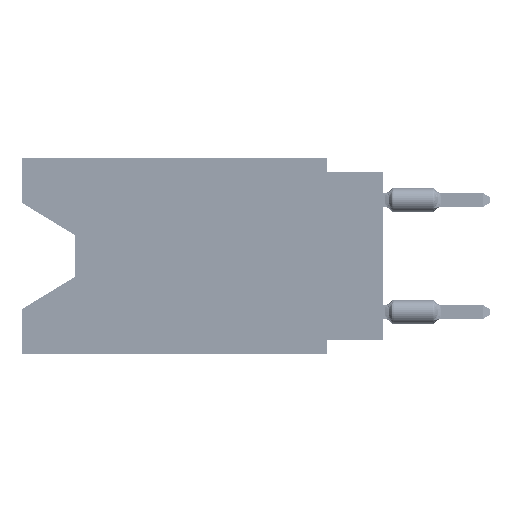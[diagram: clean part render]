
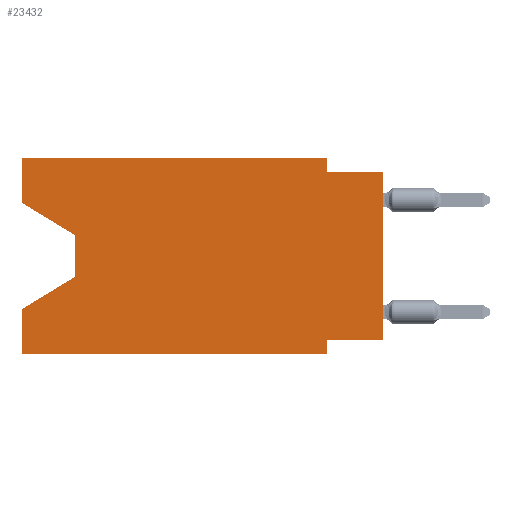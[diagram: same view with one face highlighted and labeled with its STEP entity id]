
A CAD part, left-side view. The second image highlights one B-rep face of the part: STEP entity #23432.
In plain terms, the highlighted planar face has unit normal (-1, 0, 0).
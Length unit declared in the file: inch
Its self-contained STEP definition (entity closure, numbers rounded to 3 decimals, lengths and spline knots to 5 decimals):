
#616 = EDGE_CURVE ( 'NONE', #29009, #13875, #54126, .T. ) ;
#1724 = VECTOR ( 'NONE', #10512, 39.37008 ) ;
#2000 = CARTESIAN_POINT ( 'NONE',  ( 0., 0.1, 0. ) ) ;
#3656 = CARTESIAN_POINT ( 'NONE',  ( 0., 0.645, -0.26975 ) ) ;
#3871 = LINE ( 'NONE', #20720, #44310 ) ;
#3898 = CARTESIAN_POINT ( 'NONE',  ( 0., 0.1, 0. ) ) ;
#3930 = DIRECTION ( 'NONE',  ( 0., 1., 0. ) ) ;
#5901 = LINE ( 'NONE', #15821, #15807 ) ;
#6034 = DIRECTION ( 'NONE',  ( 0., -1., 0. ) ) ;
#6709 = CARTESIAN_POINT ( 'NONE',  ( 0., 0.55, -0.212 ) ) ;
#7014 = EDGE_CURVE ( 'NONE', #55235, #61821, #58415, .T. ) ;
#7675 = EDGE_CURVE ( 'NONE', #13875, #41816, #28992, .T. ) ;
#8223 = DIRECTION ( 'NONE',  ( 0., 0., -1. ) ) ;
#9641 = EDGE_CURVE ( 'NONE', #24184, #34143, #23411, .T. ) ;
#10512 = DIRECTION ( 'NONE',  ( 0., 0., 1. ) ) ;
#11020 = ORIENTED_EDGE ( 'NONE', *, *, #616, .F. ) ;
#12656 = EDGE_CURVE ( 'NONE', #18530, #20161, #29989, .T. ) ;
#13194 = CARTESIAN_POINT ( 'NONE',  ( 0., 0.645, -0.35 ) ) ;
#13875 = VERTEX_POINT ( 'NONE', #60011 ) ;
#13877 = VERTEX_POINT ( 'NONE', #15309 ) ;
#14390 = CARTESIAN_POINT ( 'NONE',  ( 0., 0.1, -0.025 ) ) ;
#15309 = CARTESIAN_POINT ( 'NONE',  ( 0., 0.645, -0.35 ) ) ;
#15742 = EDGE_CURVE ( 'NONE', #61821, #40443, #40611, .T. ) ;
#15807 = VECTOR ( 'NONE', #71864, 39.37008 ) ;
#15821 = CARTESIAN_POINT ( 'NONE',  ( 0., 0.55, -0.212 ) ) ;
#16008 = LINE ( 'NONE', #44210, #1724 ) ;
#17539 = ORIENTED_EDGE ( 'NONE', *, *, #7014, .F. ) ;
#18102 = VECTOR ( 'NONE', #24503, 39.37008 ) ;
#18242 = CARTESIAN_POINT ( 'NONE',  ( 0., 0., -0.025 ) ) ;
#18431 = ORIENTED_EDGE ( 'NONE', *, *, #35811, .T. ) ;
#18530 = VERTEX_POINT ( 'NONE', #44497 ) ;
#19675 = CARTESIAN_POINT ( 'NONE',  ( 0., 0.645, -0.08025 ) ) ;
#20161 = VERTEX_POINT ( 'NONE', #50193 ) ;
#20720 = CARTESIAN_POINT ( 'NONE',  ( 0., 0.645, 0. ) ) ;
#21095 = ORIENTED_EDGE ( 'NONE', *, *, #34556, .T. ) ;
#22560 = ORIENTED_EDGE ( 'NONE', *, *, #15742, .F. ) ;
#23411 = LINE ( 'NONE', #57493, #18102 ) ;
#23432 = ADVANCED_FACE ( 'NONE', ( #60727 ), #44574, .F. ) ;
#24111 = CARTESIAN_POINT ( 'NONE',  ( 0., 0., -0.025 ) ) ;
#24184 = VERTEX_POINT ( 'NONE', #64884 ) ;
#24377 = VECTOR ( 'NONE', #28468, 39.37008 ) ;
#24503 = DIRECTION ( 'NONE',  ( 0., 0., -1. ) ) ;
#25063 = EDGE_CURVE ( 'NONE', #20161, #55235, #3871, .T. ) ;
#25941 = ORIENTED_EDGE ( 'NONE', *, *, #71342, .T. ) ;
#26684 = EDGE_LOOP ( 'NONE', ( #25941, #40766, #18431, #63952, #21095, #55976, #11020, #67967, #22560, #17539, #61098, #70135 ) ) ;
#27714 = CARTESIAN_POINT ( 'NONE',  ( 0., 0.645, 0. ) ) ;
#28468 = DIRECTION ( 'NONE',  ( 0., 0., 1. ) ) ;
#28992 = LINE ( 'NONE', #44786, #62373 ) ;
#29009 = VERTEX_POINT ( 'NONE', #65860 ) ;
#29989 = LINE ( 'NONE', #52366, #31119 ) ;
#30378 = CARTESIAN_POINT ( 'NONE',  ( 0., 0.1, -0.35 ) ) ;
#31119 = VECTOR ( 'NONE', #47213, 39.37008 ) ;
#33970 = LINE ( 'NONE', #67360, #24377 ) ;
#34143 = VERTEX_POINT ( 'NONE', #6709 ) ;
#34556 = EDGE_CURVE ( 'NONE', #13877, #41816, #67830, .T. ) ;
#35468 = EDGE_CURVE ( 'NONE', #29009, #40443, #16008, .T. ) ;
#35811 = EDGE_CURVE ( 'NONE', #34143, #36071, #5901, .T. ) ;
#36071 = VERTEX_POINT ( 'NONE', #3656 ) ;
#40443 = VERTEX_POINT ( 'NONE', #18242 ) ;
#40611 = LINE ( 'NONE', #24111, #44867 ) ;
#40766 = ORIENTED_EDGE ( 'NONE', *, *, #9641, .T. ) ;
#41028 = DIRECTION ( 'NONE',  ( 0., -1., 0. ) ) ;
#41816 = VERTEX_POINT ( 'NONE', #30378 ) ;
#44210 = CARTESIAN_POINT ( 'NONE',  ( 0., 0., 0. ) ) ;
#44310 = VECTOR ( 'NONE', #6034, 39.37008 ) ;
#44497 = CARTESIAN_POINT ( 'NONE',  ( 0., 0.645, -0.08025 ) ) ;
#44574 = PLANE ( 'NONE',  #54845 ) ;
#44786 = CARTESIAN_POINT ( 'NONE',  ( 0., 0.1, -0.35 ) ) ;
#44867 = VECTOR ( 'NONE', #62634, 39.37008 ) ;
#47213 = DIRECTION ( 'NONE',  ( 0., 0., 1. ) ) ;
#48002 = EDGE_CURVE ( 'NONE', #13877, #36071, #33970, .T. ) ;
#50193 = CARTESIAN_POINT ( 'NONE',  ( 0., 0.645, 0. ) ) ;
#50791 = DIRECTION ( 'NONE',  ( 0., 0., -1. ) ) ;
#51369 = VECTOR ( 'NONE', #8223, 39.37008 ) ;
#52366 = CARTESIAN_POINT ( 'NONE',  ( 0., 0.645, 0. ) ) ;
#52756 = VECTOR ( 'NONE', #3930, 39.37008 ) ;
#53101 = VECTOR ( 'NONE', #41028, 39.37008 ) ;
#54126 = LINE ( 'NONE', #55211, #52756 ) ;
#54845 = AXIS2_PLACEMENT_3D ( 'NONE', #27714, #60360, #50791 ) ;
#55211 = CARTESIAN_POINT ( 'NONE',  ( 0., 0., -0.325 ) ) ;
#55235 = VERTEX_POINT ( 'NONE', #3898 ) ;
#55976 = ORIENTED_EDGE ( 'NONE', *, *, #7675, .F. ) ;
#57493 = CARTESIAN_POINT ( 'NONE',  ( 0., 0.55, -0.138 ) ) ;
#58415 = LINE ( 'NONE', #2000, #51369 ) ;
#58877 = DIRECTION ( 'NONE',  ( 0., -0.855, -0.519 ) ) ;
#60011 = CARTESIAN_POINT ( 'NONE',  ( 0., 0.1, -0.325 ) ) ;
#60360 = DIRECTION ( 'NONE',  ( 1., 0., 0. ) ) ;
#60727 = FACE_OUTER_BOUND ( 'NONE', #26684, .T. ) ;
#61098 = ORIENTED_EDGE ( 'NONE', *, *, #25063, .F. ) ;
#61667 = DIRECTION ( 'NONE',  ( 0., 0., -1. ) ) ;
#61821 = VERTEX_POINT ( 'NONE', #14390 ) ;
#62145 = VECTOR ( 'NONE', #58877, 39.37008 ) ;
#62373 = VECTOR ( 'NONE', #61667, 39.37008 ) ;
#62634 = DIRECTION ( 'NONE',  ( 0., -1., 0. ) ) ;
#63952 = ORIENTED_EDGE ( 'NONE', *, *, #48002, .F. ) ;
#64884 = CARTESIAN_POINT ( 'NONE',  ( 0., 0.55, -0.138 ) ) ;
#65860 = CARTESIAN_POINT ( 'NONE',  ( 0., 0., -0.325 ) ) ;
#67360 = CARTESIAN_POINT ( 'NONE',  ( 0., 0.645, 0. ) ) ;
#67830 = LINE ( 'NONE', #13194, #53101 ) ;
#67967 = ORIENTED_EDGE ( 'NONE', *, *, #35468, .T. ) ;
#70135 = ORIENTED_EDGE ( 'NONE', *, *, #12656, .F. ) ;
#70592 = LINE ( 'NONE', #19675, #62145 ) ;
#71342 = EDGE_CURVE ( 'NONE', #18530, #24184, #70592, .T. ) ;
#71864 = DIRECTION ( 'NONE',  ( 0., 0.855, -0.519 ) ) ;
